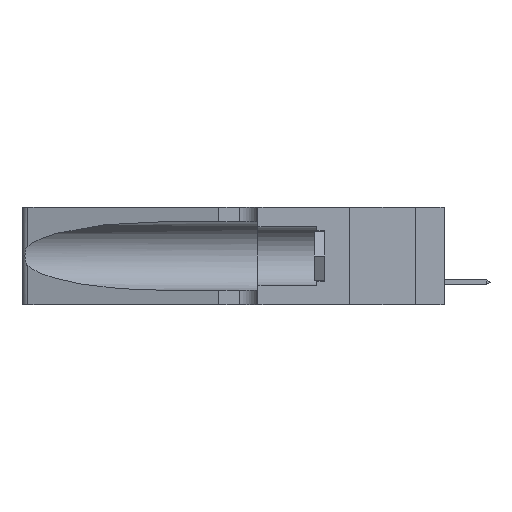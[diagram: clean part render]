
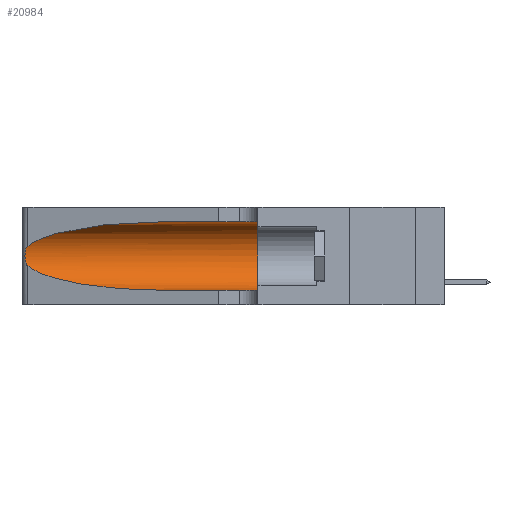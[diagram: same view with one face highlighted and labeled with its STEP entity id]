
A CAD part, left-side view. The second image highlights one B-rep face of the part: STEP entity #20984.
In plain terms, the highlighted cylindrical face has radius 3.308 mm (diameter 6.617 mm), a partial arc.
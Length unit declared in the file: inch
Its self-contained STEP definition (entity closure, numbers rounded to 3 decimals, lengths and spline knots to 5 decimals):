
#325 = CARTESIAN_POINT ( 'NONE',  ( 0.26018, 1.23835, 0.19895 ) ) ;
#548 = FACE_OUTER_BOUND ( 'NONE', #4610, .T. ) ;
#589 =( BOUNDED_CURVE ( )  B_SPLINE_CURVE ( 3, ( #32572, #25021, #25254, #9599 ),
 .UNSPECIFIED., .F., .T. ) 
 B_SPLINE_CURVE_WITH_KNOTS ( ( 4, 4 ),
 ( 1.5708, 2.84003 ),
 .UNSPECIFIED. ) 
 CURVE ( )  GEOMETRIC_REPRESENTATION_ITEM ( )  RATIONAL_B_SPLINE_CURVE ( ( 1., 0.87, 0.87, 1. ) ) 
 REPRESENTATION_ITEM ( '' )  );
#1098 = VERTEX_POINT ( 'NONE', #9306 ) ;
#1855 = LINE ( 'NONE', #4711, #26004 ) ;
#1878 = LINE ( 'NONE', #4709, #25257 ) ;
#2829 = CARTESIAN_POINT ( 'NONE',  ( 0.26075, 1.23896, 0.178 ) ) ;
#2922 = VERTEX_POINT ( 'NONE', #21241 ) ;
#2959 = CARTESIAN_POINT ( 'NONE',  ( 0.1305, 0.72297, 0.31525 ) ) ;
#4005 = CARTESIAN_POINT ( 'NONE',  ( 0.25487, 1.22718, 0.14631 ) ) ;
#4610 = EDGE_LOOP ( 'NONE', ( #19396, #18036, #21760, #20938, #11865, #30747 ) ) ;
#4709 = CARTESIAN_POINT ( 'NONE',  ( 0.1305, 1.61858, 0.05475 ) ) ;
#4711 = CARTESIAN_POINT ( 'NONE',  ( 0.1305, 1.61858, 0.31525 ) ) ;
#5108 = CARTESIAN_POINT ( 'NONE',  ( 0.25639, 1.23184, 0.21858 ) ) ;
#5526 = CARTESIAN_POINT ( 'NONE',  ( 0.25487, 1.22718, 0.14631 ) ) ;
#6186 = EDGE_CURVE ( 'NONE', #24951, #2922, #12636, .T. ) ;
#7053 = DIRECTION ( 'NONE',  ( 0., 0., 1. ) ) ;
#7065 = EDGE_CURVE ( 'NONE', #1098, #22453, #25350, .T. ) ;
#7698 = CARTESIAN_POINT ( 'NONE',  ( 0.25639, 1.23186, 0.15144 ) ) ;
#7802 = CARTESIAN_POINT ( 'NONE',  ( 0.25856, 1.23593, 0.16098 ) ) ;
#9306 = CARTESIAN_POINT ( 'NONE',  ( 0.1305, 0.35, 0.31525 ) ) ;
#9599 = CARTESIAN_POINT ( 'NONE',  ( 0.25487, 1.22718, 0.22369 ) ) ;
#10752 = CARTESIAN_POINT ( 'NONE',  ( 0.1305, 1.61858, 0.185 ) ) ;
#11865 = ORIENTED_EDGE ( 'NONE', *, *, #7065, .F. ) ;
#12212 = CARTESIAN_POINT ( 'NONE',  ( 0.1305, 0.35, 0.05475 ) ) ;
#12636 =( BOUNDED_CURVE ( )  B_SPLINE_CURVE ( 3, ( #4005, #19072, #27065, #27188 ),
 .UNSPECIFIED., .F., .T. ) 
 B_SPLINE_CURVE_WITH_KNOTS ( ( 4, 4 ),
 ( 3.44316, 4.71239 ),
 .UNSPECIFIED. ) 
 CURVE ( )  GEOMETRIC_REPRESENTATION_ITEM ( )  RATIONAL_B_SPLINE_CURVE ( ( 1., 0.87, 0.87, 1. ) ) 
 REPRESENTATION_ITEM ( '' )  );
#12689 = CARTESIAN_POINT ( 'NONE',  ( 0.25487, 1.22718, 0.22369 ) ) ;
#13282 = AXIS2_PLACEMENT_3D ( 'NONE', #22487, #29673, #7053 ) ;
#13587 = AXIS2_PLACEMENT_3D ( 'NONE', #10752, #16172, #31712 ) ;
#14579 = EDGE_CURVE ( 'NONE', #26415, #28450, #589, .T. ) ;
#15087 = DIRECTION ( 'NONE',  ( 0., -1., 0. ) ) ;
#15798 = CARTESIAN_POINT ( 'NONE',  ( 0.25555, 1.22993, 0.14849 ) ) ;
#16172 = DIRECTION ( 'NONE',  ( 0., -1., 0. ) ) ;
#18036 = ORIENTED_EDGE ( 'NONE', *, *, #29577, .T. ) ;
#19072 = CARTESIAN_POINT ( 'NONE',  ( 0.2373, 1.15595, 0.08982 ) ) ;
#19396 = ORIENTED_EDGE ( 'NONE', *, *, #14579, .T. ) ;
#20628 = CARTESIAN_POINT ( 'NONE',  ( 0.26075, 1.23896, 0.19203 ) ) ;
#20633 = EDGE_CURVE ( 'NONE', #2922, #22453, #1878, .T. ) ;
#20938 = ORIENTED_EDGE ( 'NONE', *, *, #20633, .T. ) ;
#20949 = CARTESIAN_POINT ( 'NONE',  ( 0.25789, 1.23486, 0.15765 ) ) ;
#20984 = ADVANCED_FACE ( 'NONE', ( #548 ), #23132, .F. ) ;
#21241 = CARTESIAN_POINT ( 'NONE',  ( 0.1305, 0.72297, 0.05475 ) ) ;
#21760 = ORIENTED_EDGE ( 'NONE', *, *, #6186, .T. ) ;
#22453 = VERTEX_POINT ( 'NONE', #12212 ) ;
#22487 = CARTESIAN_POINT ( 'NONE',  ( 0.1305, 0.35, 0.185 ) ) ;
#23132 = CYLINDRICAL_SURFACE ( 'NONE', #13587, 0.13025 ) ;
#23343 = CARTESIAN_POINT ( 'NONE',  ( 0.25787, 1.23484, 0.2124 ) ) ;
#24951 = VERTEX_POINT ( 'NONE', #26130 ) ;
#25021 = CARTESIAN_POINT ( 'NONE',  ( 0.18966, 0.96281, 0.31525 ) ) ;
#25254 = CARTESIAN_POINT ( 'NONE',  ( 0.2373, 1.15595, 0.28018 ) ) ;
#25257 = VECTOR ( 'NONE', #33026, 39.37008 ) ;
#25350 = CIRCLE ( 'NONE', #13282, 0.13025 ) ;
#26004 = VECTOR ( 'NONE', #15087, 39.37008 ) ;
#26130 = CARTESIAN_POINT ( 'NONE',  ( 0.25487, 1.22718, 0.14631 ) ) ;
#26415 = VERTEX_POINT ( 'NONE', #2959 ) ;
#26828 = B_SPLINE_CURVE_WITH_KNOTS ( 'NONE', 3,
 ( #12689, #33295, #5108, #23343, #31207, #325, #20628, #2829, #28501, #7802, #20949, #7698, #15798, #5526 ),
 .UNSPECIFIED., .F., .F.,
 ( 4, 2, 2, 2, 2, 2, 4 ),
 ( 0., 0.00027, 0.00053, 0.00107, 0.0016, 0.00187, 0.00214 ),
 .UNSPECIFIED. ) ;
#27065 = CARTESIAN_POINT ( 'NONE',  ( 0.18966, 0.96281, 0.05475 ) ) ;
#27188 = CARTESIAN_POINT ( 'NONE',  ( 0.1305, 0.72297, 0.05475 ) ) ;
#28450 = VERTEX_POINT ( 'NONE', #31804 ) ;
#28501 = CARTESIAN_POINT ( 'NONE',  ( 0.26017, 1.23833, 0.17102 ) ) ;
#29577 = EDGE_CURVE ( 'NONE', #28450, #24951, #26828, .T. ) ;
#29673 = DIRECTION ( 'NONE',  ( 0., 1., 0. ) ) ;
#30747 = ORIENTED_EDGE ( 'NONE', *, *, #32418, .F. ) ;
#31207 = CARTESIAN_POINT ( 'NONE',  ( 0.25854, 1.2359, 0.20912 ) ) ;
#31712 = DIRECTION ( 'NONE',  ( 0., 0., -1. ) ) ;
#31804 = CARTESIAN_POINT ( 'NONE',  ( 0.25487, 1.22718, 0.22369 ) ) ;
#32418 = EDGE_CURVE ( 'NONE', #26415, #1098, #1855, .T. ) ;
#32572 = CARTESIAN_POINT ( 'NONE',  ( 0.1305, 0.72297, 0.31525 ) ) ;
#33026 = DIRECTION ( 'NONE',  ( 0., -1., 0. ) ) ;
#33295 = CARTESIAN_POINT ( 'NONE',  ( 0.25555, 1.22994, 0.2215 ) ) ;
